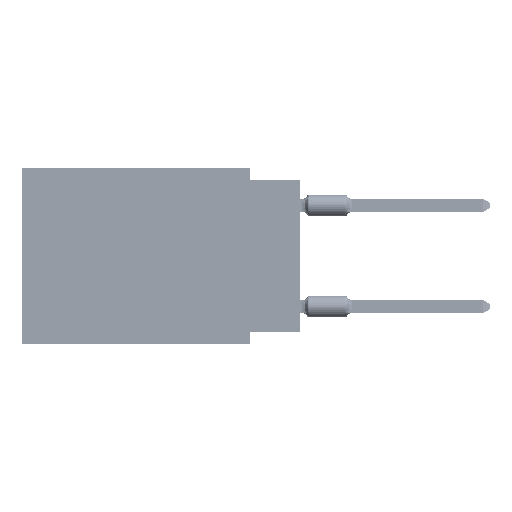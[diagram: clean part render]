
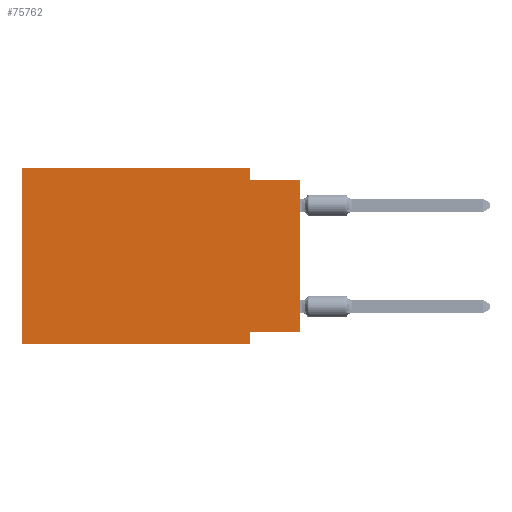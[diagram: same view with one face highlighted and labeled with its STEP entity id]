
A CAD part, left-side view. The second image highlights one B-rep face of the part: STEP entity #75762.
In plain terms, the highlighted planar face has unit normal (-1, 0, 0).
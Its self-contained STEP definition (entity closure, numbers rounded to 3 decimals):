
#580 = CARTESIAN_POINT ( 'NONE',  ( 0., 0., -8.255 ) ) ;
#734 = VERTEX_POINT ( 'NONE', #42602 ) ;
#3324 = CARTESIAN_POINT ( 'NONE',  ( 0., 13.97, -8.89 ) ) ;
#3480 = CARTESIAN_POINT ( 'NONE',  ( 0., 0., -0.635 ) ) ;
#4012 = VERTEX_POINT ( 'NONE', #83646 ) ;
#6810 = VERTEX_POINT ( 'NONE', #34171 ) ;
#9451 = CARTESIAN_POINT ( 'NONE',  ( 0., 2.54, -8.89 ) ) ;
#10089 = LINE ( 'NONE', #3324, #51580 ) ;
#11132 = DIRECTION ( 'NONE',  ( 0., -1., 0. ) ) ;
#12458 = VECTOR ( 'NONE', #56222, 1000. ) ;
#12537 = ORIENTED_EDGE ( 'NONE', *, *, #33417, .F. ) ;
#15557 = VERTEX_POINT ( 'NONE', #580 ) ;
#16344 = CARTESIAN_POINT ( 'NONE',  ( 0., 13.97, 0. ) ) ;
#18926 = VECTOR ( 'NONE', #75914, 1000. ) ;
#21519 = CARTESIAN_POINT ( 'NONE',  ( 0., 13.97, -8.89 ) ) ;
#22061 = AXIS2_PLACEMENT_3D ( 'NONE', #16344, #23569, #72781 ) ;
#22165 = CARTESIAN_POINT ( 'NONE',  ( 0., 0., -8.255 ) ) ;
#22492 = CARTESIAN_POINT ( 'NONE',  ( 0., 0., 0. ) ) ;
#23350 = DIRECTION ( 'NONE',  ( 0., 0., 1. ) ) ;
#23569 = DIRECTION ( 'NONE',  ( 1., 0., 0. ) ) ;
#28678 = VECTOR ( 'NONE', #11132, 1000. ) ;
#29373 = ORIENTED_EDGE ( 'NONE', *, *, #52464, .F. ) ;
#29915 = VECTOR ( 'NONE', #37368, 1000. ) ;
#30573 = LINE ( 'NONE', #44135, #29915 ) ;
#33065 = ORIENTED_EDGE ( 'NONE', *, *, #66684, .F. ) ;
#33417 = EDGE_CURVE ( 'NONE', #72588, #734, #45876, .T. ) ;
#34171 = CARTESIAN_POINT ( 'NONE',  ( 0., 2.54, -8.89 ) ) ;
#37368 = DIRECTION ( 'NONE',  ( 0., 0., 1. ) ) ;
#37614 = DIRECTION ( 'NONE',  ( 0., -1., 0. ) ) ;
#40395 = LINE ( 'NONE', #81944, #46313 ) ;
#41545 = VERTEX_POINT ( 'NONE', #57664 ) ;
#42602 = CARTESIAN_POINT ( 'NONE',  ( 0., 0., -0.635 ) ) ;
#44135 = CARTESIAN_POINT ( 'NONE',  ( 0., 13.97, 0. ) ) ;
#45876 = LINE ( 'NONE', #3480, #28678 ) ;
#46313 = VECTOR ( 'NONE', #88268, 1000. ) ;
#47720 = EDGE_CURVE ( 'NONE', #76270, #50186, #30573, .T. ) ;
#50186 = VERTEX_POINT ( 'NONE', #89203 ) ;
#51580 = VECTOR ( 'NONE', #37614, 1000. ) ;
#51781 = EDGE_CURVE ( 'NONE', #15557, #734, #78453, .T. ) ;
#51875 = DIRECTION ( 'NONE',  ( 0., 0., -1. ) ) ;
#52464 = EDGE_CURVE ( 'NONE', #15557, #41545, #63268, .T. ) ;
#56222 = DIRECTION ( 'NONE',  ( 0., -1., 0. ) ) ;
#57664 = CARTESIAN_POINT ( 'NONE',  ( 0., 2.54, -8.255 ) ) ;
#59029 = ORIENTED_EDGE ( 'NONE', *, *, #78135, .T. ) ;
#59435 = VECTOR ( 'NONE', #51875, 1000. ) ;
#63268 = LINE ( 'NONE', #22165, #18926 ) ;
#63443 = CARTESIAN_POINT ( 'NONE',  ( 0., 13.97, 0. ) ) ;
#64984 = LINE ( 'NONE', #9451, #59435 ) ;
#66000 = PLANE ( 'NONE',  #22061 ) ;
#66684 = EDGE_CURVE ( 'NONE', #50186, #4012, #70648, .T. ) ;
#70648 = LINE ( 'NONE', #63443, #12458 ) ;
#71379 = ORIENTED_EDGE ( 'NONE', *, *, #85642, .F. ) ;
#72588 = VERTEX_POINT ( 'NONE', #87379 ) ;
#72781 = DIRECTION ( 'NONE',  ( 0., 0., -1. ) ) ;
#73646 = VECTOR ( 'NONE', #23350, 1000. ) ;
#75762 = ADVANCED_FACE ( 'NONE', ( #85410 ), #66000, .F. ) ;
#75914 = DIRECTION ( 'NONE',  ( 0., 1., 0. ) ) ;
#76270 = VERTEX_POINT ( 'NONE', #21519 ) ;
#77355 = ORIENTED_EDGE ( 'NONE', *, *, #51781, .T. ) ;
#78135 = EDGE_CURVE ( 'NONE', #76270, #6810, #10089, .T. ) ;
#78453 = LINE ( 'NONE', #22492, #73646 ) ;
#79842 = ORIENTED_EDGE ( 'NONE', *, *, #47720, .F. ) ;
#81944 = CARTESIAN_POINT ( 'NONE',  ( 0., 2.54, 0. ) ) ;
#83646 = CARTESIAN_POINT ( 'NONE',  ( 0., 2.54, 0. ) ) ;
#84373 = EDGE_CURVE ( 'NONE', #4012, #72588, #40395, .T. ) ;
#85410 = FACE_OUTER_BOUND ( 'NONE', #86784, .T. ) ;
#85642 = EDGE_CURVE ( 'NONE', #41545, #6810, #64984, .T. ) ;
#86784 = EDGE_LOOP ( 'NONE', ( #77355, #12537, #88251, #33065, #79842, #59029, #71379, #29373 ) ) ;
#87379 = CARTESIAN_POINT ( 'NONE',  ( 0., 2.54, -0.635 ) ) ;
#88251 = ORIENTED_EDGE ( 'NONE', *, *, #84373, .F. ) ;
#88268 = DIRECTION ( 'NONE',  ( 0., 0., -1. ) ) ;
#89203 = CARTESIAN_POINT ( 'NONE',  ( 0., 13.97, 0. ) ) ;
